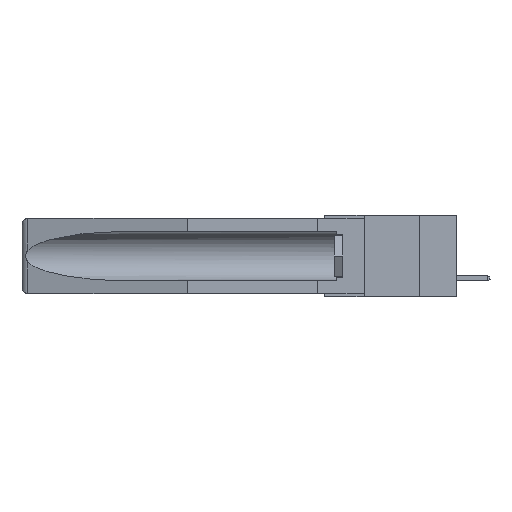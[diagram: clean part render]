
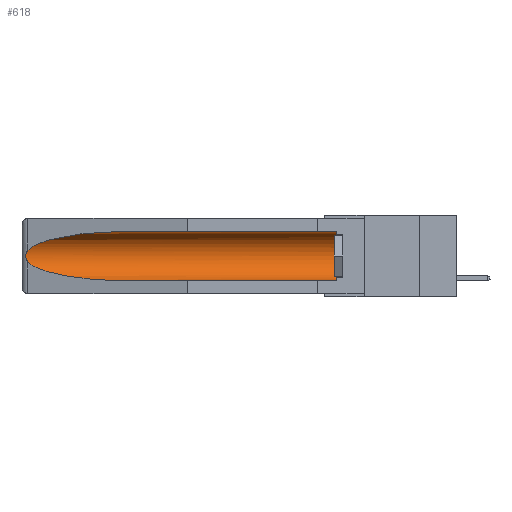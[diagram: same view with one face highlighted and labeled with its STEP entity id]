
A CAD part, left-side view. The second image highlights one B-rep face of the part: STEP entity #618.
In plain terms, the highlighted cylindrical face has radius 2.857 mm (diameter 5.715 mm), a partial arc.
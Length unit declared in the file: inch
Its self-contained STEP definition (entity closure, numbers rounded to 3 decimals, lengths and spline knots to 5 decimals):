
#45 = CARTESIAN_POINT ( 'NONE',  ( 0.2675, 1.53308, -0.16763 ) ) ;
#248 = EDGE_CURVE ( 'NONE', #10947, #6556, #11617, .T. ) ;
#293 = CARTESIAN_POINT ( 'NONE',  ( 0.26537, 1.52718, -0.19328 ) ) ;
#419 = EDGE_CURVE ( 'NONE', #8864, #6458, #7455, .T. ) ;
#618 = ADVANCED_FACE ( 'NONE', ( #8986 ), #12864, .F. ) ;
#743 = EDGE_CURVE ( 'NONE', #8864, #13861, #7645, .T. ) ;
#854 = CARTESIAN_POINT ( 'NONE',  ( 0.155, 0.126, -0.1715 ) ) ;
#973 = CARTESIAN_POINT ( 'NONE',  ( 0.155, 1.07973, -0.059 ) ) ;
#1191 = CARTESIAN_POINT ( 'NONE',  ( 0.25451, 1.48313, -0.24835 ) ) ;
#1357 = ORIENTED_EDGE ( 'NONE', *, *, #8291, .T. ) ;
#1373 = CARTESIAN_POINT ( 'NONE',  ( 0.26537, 1.52718, -0.14972 ) ) ;
#2197 = EDGE_LOOP ( 'NONE', ( #9189, #7503, #6281, #9504, #8648, #1357 ) ) ;
#2294 = CARTESIAN_POINT ( 'NONE',  ( 0.26537, 1.52718, -0.19328 ) ) ;
#2390 = CARTESIAN_POINT ( 'NONE',  ( 0.26597, 1.52961, -0.15275 ) ) ;
#2991 = CARTESIAN_POINT ( 'NONE',  ( 0.155, -0.30754, -0.1715 ) ) ;
#3445 = CARTESIAN_POINT ( 'NONE',  ( 0.21114, 1.30732, -0.284 ) ) ;
#3577 = LINE ( 'NONE', #5762, #5434 ) ;
#4255 = AXIS2_PLACEMENT_3D ( 'NONE', #854, #9224, #5489 ) ;
#5236 = EDGE_CURVE ( 'NONE', #6894, #10947, #12769, .T. ) ;
#5312 = EDGE_CURVE ( 'NONE', #6556, #6458, #6570, .T. ) ;
#5434 = VECTOR ( 'NONE', #10477, 39.37008 ) ;
#5489 = DIRECTION ( 'NONE',  ( 0., 0., 1. ) ) ;
#5528 = CARTESIAN_POINT ( 'NONE',  ( 0.25451, 1.48313, -0.09465 ) ) ;
#5762 = CARTESIAN_POINT ( 'NONE',  ( 0.155, -0.30754, -0.059 ) ) ;
#5815 = CARTESIAN_POINT ( 'NONE',  ( 0.155, -0.30754, -0.284 ) ) ;
#5962 = CARTESIAN_POINT ( 'NONE',  ( 0.26537, 1.52718, -0.14972 ) ) ;
#6281 = ORIENTED_EDGE ( 'NONE', *, *, #5312, .T. ) ;
#6458 = VERTEX_POINT ( 'NONE', #14619 ) ;
#6556 = VERTEX_POINT ( 'NONE', #293 ) ;
#6570 =( BOUNDED_CURVE ( )  B_SPLINE_CURVE ( 3, ( #2294, #1191, #3445, #10617 ),
 .UNSPECIFIED., .F., .T. ) 
 B_SPLINE_CURVE_WITH_KNOTS ( ( 4, 4 ),
 ( 0.1948, 1.5708 ),
 .UNSPECIFIED. ) 
 CURVE ( )  GEOMETRIC_REPRESENTATION_ITEM ( )  RATIONAL_B_SPLINE_CURVE ( ( 1., 0.848, 0.848, 1. ) ) 
 REPRESENTATION_ITEM ( '' )  );
#6856 = CARTESIAN_POINT ( 'NONE',  ( 0.26537, 1.52718, -0.14972 ) ) ;
#6894 = VERTEX_POINT ( 'NONE', #973 ) ;
#7370 = CARTESIAN_POINT ( 'NONE',  ( 0.155, 0.126, -0.059 ) ) ;
#7455 = LINE ( 'NONE', #5815, #12116 ) ;
#7503 = ORIENTED_EDGE ( 'NONE', *, *, #248, .T. ) ;
#7645 = CIRCLE ( 'NONE', #4255, 0.1125 ) ;
#7921 = CARTESIAN_POINT ( 'NONE',  ( 0.21114, 1.30732, -0.059 ) ) ;
#8175 = DIRECTION ( 'NONE',  ( 0., 1., 0. ) ) ;
#8249 = AXIS2_PLACEMENT_3D ( 'NONE', #2991, #14742, #8815 ) ;
#8274 = CARTESIAN_POINT ( 'NONE',  ( 0.2673, 1.5327, -0.16383 ) ) ;
#8291 = EDGE_CURVE ( 'NONE', #13861, #6894, #3577, .T. ) ;
#8648 = ORIENTED_EDGE ( 'NONE', *, *, #743, .T. ) ;
#8815 = DIRECTION ( 'NONE',  ( 0., 0., 1. ) ) ;
#8864 = VERTEX_POINT ( 'NONE', #13960 ) ;
#8986 = FACE_OUTER_BOUND ( 'NONE', #2197, .T. ) ;
#9189 = ORIENTED_EDGE ( 'NONE', *, *, #5236, .T. ) ;
#9224 = DIRECTION ( 'NONE',  ( 0., -1., 0. ) ) ;
#9375 = CARTESIAN_POINT ( 'NONE',  ( 0.26655, 1.53094, -0.18657 ) ) ;
#9504 = ORIENTED_EDGE ( 'NONE', *, *, #419, .F. ) ;
#10477 = DIRECTION ( 'NONE',  ( 0., 1., 0. ) ) ;
#10617 = CARTESIAN_POINT ( 'NONE',  ( 0.155, 1.07973, -0.284 ) ) ;
#10770 = CARTESIAN_POINT ( 'NONE',  ( 0.2675, 1.53308, -0.17534 ) ) ;
#10947 = VERTEX_POINT ( 'NONE', #1373 ) ;
#11617 = B_SPLINE_CURVE_WITH_KNOTS ( 'NONE', 3,
 ( #5962, #2390, #14343, #8274, #45, #10770, #11783, #9375, #11726, #12943 ),
 .UNSPECIFIED., .F., .F.,
 ( 4, 2, 2, 2, 4 ),
 ( 0., 0.00029, 0.00058, 0.00087, 0.00117 ),
 .UNSPECIFIED. ) ;
#11726 = CARTESIAN_POINT ( 'NONE',  ( 0.26597, 1.5296, -0.19026 ) ) ;
#11783 = CARTESIAN_POINT ( 'NONE',  ( 0.2673, 1.53269, -0.17917 ) ) ;
#12116 = VECTOR ( 'NONE', #8175, 39.37008 ) ;
#12769 =( BOUNDED_CURVE ( )  B_SPLINE_CURVE ( 3, ( #15088, #7921, #5528, #6856 ),
 .UNSPECIFIED., .F., .T. ) 
 B_SPLINE_CURVE_WITH_KNOTS ( ( 4, 4 ),
 ( 4.71239, 6.08839 ),
 .UNSPECIFIED. ) 
 CURVE ( )  GEOMETRIC_REPRESENTATION_ITEM ( )  RATIONAL_B_SPLINE_CURVE ( ( 1., 0.848, 0.848, 1. ) ) 
 REPRESENTATION_ITEM ( '' )  );
#12864 = CYLINDRICAL_SURFACE ( 'NONE', #8249, 0.1125 ) ;
#12943 = CARTESIAN_POINT ( 'NONE',  ( 0.26537, 1.52718, -0.19328 ) ) ;
#13861 = VERTEX_POINT ( 'NONE', #7370 ) ;
#13960 = CARTESIAN_POINT ( 'NONE',  ( 0.155, 0.126, -0.284 ) ) ;
#14343 = CARTESIAN_POINT ( 'NONE',  ( 0.26654, 1.53092, -0.15636 ) ) ;
#14619 = CARTESIAN_POINT ( 'NONE',  ( 0.155, 1.07973, -0.284 ) ) ;
#14742 = DIRECTION ( 'NONE',  ( 0., 1., 0. ) ) ;
#15088 = CARTESIAN_POINT ( 'NONE',  ( 0.155, 1.07973, -0.059 ) ) ;
